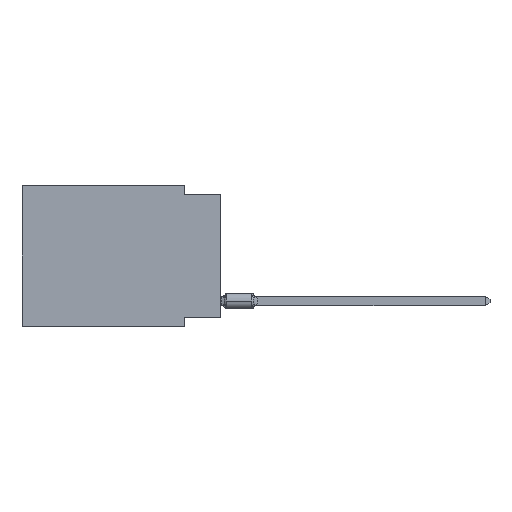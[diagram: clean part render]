
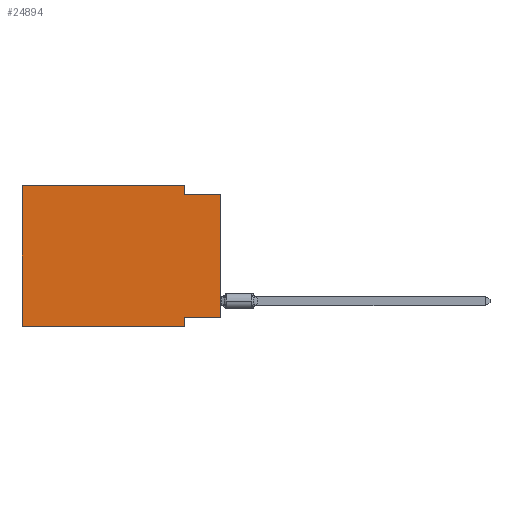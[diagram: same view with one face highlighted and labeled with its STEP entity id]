
A CAD part, left-side view. The second image highlights one B-rep face of the part: STEP entity #24894.
In plain terms, the highlighted planar face has unit normal (-1, 0, 0).
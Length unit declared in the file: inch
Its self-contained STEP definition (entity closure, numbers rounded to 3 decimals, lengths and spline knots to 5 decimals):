
#155 = DIRECTION ( 'NONE',  ( 0., 0., 1. ) ) ;
#322 = EDGE_CURVE ( 'NONE', #19259, #5863, #56599, .T. ) ;
#2344 = CARTESIAN_POINT ( 'NONE',  ( 0., 0.1, -0.39 ) ) ;
#2451 = CARTESIAN_POINT ( 'NONE',  ( 0., 0.55, -0.39 ) ) ;
#3951 = VECTOR ( 'NONE', #17609, 39.37008 ) ;
#4636 = CARTESIAN_POINT ( 'NONE',  ( 0., 0., -0.025 ) ) ;
#5018 = DIRECTION ( 'NONE',  ( 0., 0., -1. ) ) ;
#5172 = FACE_OUTER_BOUND ( 'NONE', #71122, .T. ) ;
#5658 = CARTESIAN_POINT ( 'NONE',  ( 0., 0., -0.365 ) ) ;
#5863 = VERTEX_POINT ( 'NONE', #63922 ) ;
#6111 = ORIENTED_EDGE ( 'NONE', *, *, #18100, .F. ) ;
#8354 = ORIENTED_EDGE ( 'NONE', *, *, #59881, .F. ) ;
#9588 = EDGE_CURVE ( 'NONE', #71958, #46362, #82812, .T. ) ;
#10709 = VECTOR ( 'NONE', #155, 39.37008 ) ;
#12307 = CARTESIAN_POINT ( 'NONE',  ( 0., 0., -0.025 ) ) ;
#16677 = ORIENTED_EDGE ( 'NONE', *, *, #70190, .T. ) ;
#17609 = DIRECTION ( 'NONE',  ( 0., 1., 0. ) ) ;
#18100 = EDGE_CURVE ( 'NONE', #73452, #33098, #69461, .T. ) ;
#18559 = DIRECTION ( 'NONE',  ( 1., 0., 0. ) ) ;
#19259 = VERTEX_POINT ( 'NONE', #22421 ) ;
#19461 = VECTOR ( 'NONE', #29207, 39.37008 ) ;
#22421 = CARTESIAN_POINT ( 'NONE',  ( 0., 0.55, 0. ) ) ;
#23377 = CARTESIAN_POINT ( 'NONE',  ( 0., 0.55, 0. ) ) ;
#24553 = DIRECTION ( 'NONE',  ( 0., 0., -1. ) ) ;
#24889 = LINE ( 'NONE', #62897, #58495 ) ;
#24894 = ADVANCED_FACE ( 'NONE', ( #5172 ), #77740, .F. ) ;
#25168 = CARTESIAN_POINT ( 'NONE',  ( 0., 0.55, 0. ) ) ;
#28783 = LINE ( 'NONE', #25168, #19461 ) ;
#28784 = DIRECTION ( 'NONE',  ( 0., -1., 0. ) ) ;
#29207 = DIRECTION ( 'NONE',  ( 0., 0., 1. ) ) ;
#32141 = VECTOR ( 'NONE', #43073, 39.37008 ) ;
#33098 = VERTEX_POINT ( 'NONE', #35933 ) ;
#34664 = LINE ( 'NONE', #67074, #10709 ) ;
#35262 = LINE ( 'NONE', #2451, #45136 ) ;
#35933 = CARTESIAN_POINT ( 'NONE',  ( 0., 0.1, -0.365 ) ) ;
#36280 = DIRECTION ( 'NONE',  ( 0., 0., -1. ) ) ;
#39815 = CARTESIAN_POINT ( 'NONE',  ( 0., 0.1, -0.025 ) ) ;
#43073 = DIRECTION ( 'NONE',  ( 0., -1., 0. ) ) ;
#43362 = ORIENTED_EDGE ( 'NONE', *, *, #82728, .F. ) ;
#43611 = CARTESIAN_POINT ( 'NONE',  ( 0., 0.55, 0. ) ) ;
#44056 = ORIENTED_EDGE ( 'NONE', *, *, #74482, .F. ) ;
#45136 = VECTOR ( 'NONE', #28784, 39.37008 ) ;
#46362 = VERTEX_POINT ( 'NONE', #12307 ) ;
#46651 = VERTEX_POINT ( 'NONE', #2344 ) ;
#56599 = LINE ( 'NONE', #23377, #78187 ) ;
#57276 = ORIENTED_EDGE ( 'NONE', *, *, #81349, .T. ) ;
#58495 = VECTOR ( 'NONE', #5018, 39.37008 ) ;
#58733 = AXIS2_PLACEMENT_3D ( 'NONE', #43611, #18559, #36280 ) ;
#59881 = EDGE_CURVE ( 'NONE', #5863, #71958, #24889, .T. ) ;
#62646 = DIRECTION ( 'NONE',  ( 0., -1., 0. ) ) ;
#62897 = CARTESIAN_POINT ( 'NONE',  ( 0., 0.1, 0. ) ) ;
#63922 = CARTESIAN_POINT ( 'NONE',  ( 0., 0.1, 0. ) ) ;
#64911 = ORIENTED_EDGE ( 'NONE', *, *, #322, .F. ) ;
#67074 = CARTESIAN_POINT ( 'NONE',  ( 0., 0., 0. ) ) ;
#69461 = LINE ( 'NONE', #84083, #3951 ) ;
#70190 = EDGE_CURVE ( 'NONE', #76179, #46651, #35262, .T. ) ;
#70357 = LINE ( 'NONE', #83694, #72747 ) ;
#71122 = EDGE_LOOP ( 'NONE', ( #57276, #77064, #8354, #64911, #44056, #16677, #43362, #6111 ) ) ;
#71958 = VERTEX_POINT ( 'NONE', #39815 ) ;
#72747 = VECTOR ( 'NONE', #24553, 39.37008 ) ;
#73452 = VERTEX_POINT ( 'NONE', #5658 ) ;
#74482 = EDGE_CURVE ( 'NONE', #76179, #19259, #28783, .T. ) ;
#76179 = VERTEX_POINT ( 'NONE', #81807 ) ;
#77064 = ORIENTED_EDGE ( 'NONE', *, *, #9588, .F. ) ;
#77740 = PLANE ( 'NONE',  #58733 ) ;
#78187 = VECTOR ( 'NONE', #62646, 39.37008 ) ;
#81349 = EDGE_CURVE ( 'NONE', #73452, #46362, #34664, .T. ) ;
#81807 = CARTESIAN_POINT ( 'NONE',  ( 0., 0.55, -0.39 ) ) ;
#82728 = EDGE_CURVE ( 'NONE', #33098, #46651, #70357, .T. ) ;
#82812 = LINE ( 'NONE', #4636, #32141 ) ;
#83694 = CARTESIAN_POINT ( 'NONE',  ( 0., 0.1, -0.39 ) ) ;
#84083 = CARTESIAN_POINT ( 'NONE',  ( 0., 0., -0.365 ) ) ;
